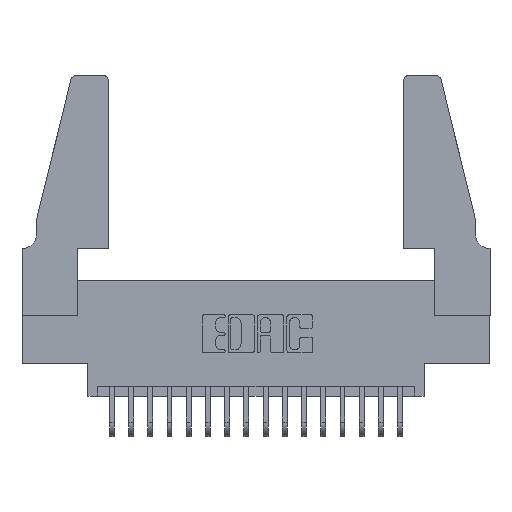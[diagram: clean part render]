
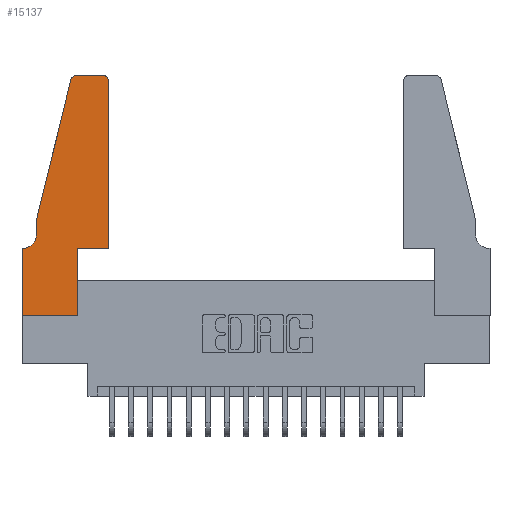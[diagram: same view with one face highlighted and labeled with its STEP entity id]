
A CAD part, top view. The second image highlights one B-rep face of the part: STEP entity #15137.
In plain terms, the highlighted planar face has unit normal (0, 0, 1).
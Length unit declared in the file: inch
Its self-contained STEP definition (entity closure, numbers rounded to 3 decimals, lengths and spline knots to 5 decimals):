
#219 = DIRECTION ( 'NONE',  ( 0., 0., 1. ) ) ;
#466 = EDGE_LOOP ( 'NONE', ( #16806, #18233, #15224, #2376, #16468, #2192, #2934, #1054, #9413, #13160, #19247, #13329 ) ) ;
#590 = VERTEX_POINT ( 'NONE', #2624 ) ;
#904 = AXIS2_PLACEMENT_3D ( 'NONE', #11156, #1846, #12693 ) ;
#1036 = DIRECTION ( 'NONE',  ( -0.239, -0.971, 0. ) ) ;
#1054 = ORIENTED_EDGE ( 'NONE', *, *, #2095, .T. ) ;
#1112 = EDGE_CURVE ( 'NONE', #2740, #590, #12800, .T. ) ;
#1832 = VERTEX_POINT ( 'NONE', #8093 ) ;
#1846 = DIRECTION ( 'NONE',  ( 0., 0., 1. ) ) ;
#1864 = LINE ( 'NONE', #18925, #17816 ) ;
#1996 = CARTESIAN_POINT ( 'NONE',  ( 0.0055, 0.42, 0.37 ) ) ;
#2095 = EDGE_CURVE ( 'NONE', #8493, #2740, #3564, .T. ) ;
#2192 = ORIENTED_EDGE ( 'NONE', *, *, #6867, .T. ) ;
#2376 = ORIENTED_EDGE ( 'NONE', *, *, #12319, .T. ) ;
#2624 = CARTESIAN_POINT ( 'NONE',  ( 0.2865, 0.35, 0.37 ) ) ;
#2740 = VERTEX_POINT ( 'NONE', #13119 ) ;
#2934 = ORIENTED_EDGE ( 'NONE', *, *, #7470, .T. ) ;
#3076 = CARTESIAN_POINT ( 'NONE',  ( 0.0755, 0.5, 0.37 ) ) ;
#3233 = DIRECTION ( 'NONE',  ( 0., 1., 0. ) ) ;
#3564 = LINE ( 'NONE', #8629, #16355 ) ;
#3566 = DIRECTION ( 'NONE',  ( -1., 0., 0. ) ) ;
#3682 = CARTESIAN_POINT ( 'NONE',  ( 0.0755, 0.35, 0.37 ) ) ;
#4038 = VERTEX_POINT ( 'NONE', #10125 ) ;
#4197 = CARTESIAN_POINT ( 'NONE',  ( 0.0755, 0.5, 0.37 ) ) ;
#4335 = CARTESIAN_POINT ( 'NONE',  ( 0., 0., 0.37 ) ) ;
#5268 = DIRECTION ( 'NONE',  ( -1., 0., 0. ) ) ;
#5428 = AXIS2_PLACEMENT_3D ( 'NONE', #6607, #17380, #8152 ) ;
#5600 = VECTOR ( 'NONE', #6764, 39.37008 ) ;
#5703 = VECTOR ( 'NONE', #7060, 39.37008 ) ;
#6096 = LINE ( 'NONE', #19104, #5600 ) ;
#6125 = EDGE_CURVE ( 'NONE', #7787, #16959, #12866, .T. ) ;
#6607 = CARTESIAN_POINT ( 'NONE',  ( 0.4205, 1.22, 0.37 ) ) ;
#6764 = DIRECTION ( 'NONE',  ( 0., 1., 0. ) ) ;
#6867 = EDGE_CURVE ( 'NONE', #16959, #18487, #9449, .T. ) ;
#7060 = DIRECTION ( 'NONE',  ( -1., 0., 0. ) ) ;
#7470 = EDGE_CURVE ( 'NONE', #18487, #8493, #1864, .T. ) ;
#7595 = CARTESIAN_POINT ( 'NONE',  ( 0.4505, 0.35, 0.37 ) ) ;
#7738 = LINE ( 'NONE', #16715, #11854 ) ;
#7787 = VERTEX_POINT ( 'NONE', #16619 ) ;
#8093 = CARTESIAN_POINT ( 'NONE',  ( 0.4205, 1.25, 0.37 ) ) ;
#8152 = DIRECTION ( 'NONE',  ( 1., 0., 0. ) ) ;
#8429 = EDGE_CURVE ( 'NONE', #13357, #12403, #13708, .T. ) ;
#8493 = VERTEX_POINT ( 'NONE', #4335 ) ;
#8629 = CARTESIAN_POINT ( 'NONE',  ( 0., 0., 0.37 ) ) ;
#9413 = ORIENTED_EDGE ( 'NONE', *, *, #1112, .T. ) ;
#9449 = LINE ( 'NONE', #3682, #9927 ) ;
#9527 = EDGE_CURVE ( 'NONE', #1832, #12207, #10296, .T. ) ;
#9563 = CIRCLE ( 'NONE', #5428, 0.03 ) ;
#9927 = VECTOR ( 'NONE', #5268, 39.37008 ) ;
#10018 = CARTESIAN_POINT ( 'NONE',  ( 0.4505, 0.35, 0.37 ) ) ;
#10125 = CARTESIAN_POINT ( 'NONE',  ( 0.4505, 1.22, 0.37 ) ) ;
#10186 = CARTESIAN_POINT ( 'NONE',  ( 0.2605, 1.25, 0.37 ) ) ;
#10203 = DIRECTION ( 'NONE',  ( 1., 0., 0. ) ) ;
#10296 = LINE ( 'NONE', #10186, #5703 ) ;
#11008 = CARTESIAN_POINT ( 'NONE',  ( 0., 0.35, 0.37 ) ) ;
#11072 = DIRECTION ( 'NONE',  ( 1., 0., 0. ) ) ;
#11156 = CARTESIAN_POINT ( 'NONE',  ( 0.284, 1.22, 0.37 ) ) ;
#11550 = DIRECTION ( 'NONE',  ( 1., 0., 0. ) ) ;
#11854 = VECTOR ( 'NONE', #18319, 39.37008 ) ;
#12122 = FACE_OUTER_BOUND ( 'NONE', #466, .T. ) ;
#12207 = VERTEX_POINT ( 'NONE', #13417 ) ;
#12319 = EDGE_CURVE ( 'NONE', #12403, #7787, #7738, .T. ) ;
#12325 = VECTOR ( 'NONE', #3233, 39.37008 ) ;
#12341 = CARTESIAN_POINT ( 'NONE',  ( 0., 0.35, 0.37 ) ) ;
#12403 = VERTEX_POINT ( 'NONE', #3076 ) ;
#12693 = DIRECTION ( 'NONE',  ( 1., 0., 0. ) ) ;
#12800 = LINE ( 'NONE', #14103, #12325 ) ;
#12802 = DIRECTION ( 'NONE',  ( 0., -1., 0. ) ) ;
#12834 = DIRECTION ( 'NONE',  ( 0., 0., -1. ) ) ;
#12866 = CIRCLE ( 'NONE', #18377, 0.07 ) ;
#13119 = CARTESIAN_POINT ( 'NONE',  ( 0.2865, 0., 0.37 ) ) ;
#13160 = ORIENTED_EDGE ( 'NONE', *, *, #19455, .T. ) ;
#13221 = EDGE_CURVE ( 'NONE', #4038, #1832, #9563, .T. ) ;
#13329 = ORIENTED_EDGE ( 'NONE', *, *, #13221, .T. ) ;
#13357 = VERTEX_POINT ( 'NONE', #19198 ) ;
#13417 = CARTESIAN_POINT ( 'NONE',  ( 0.284, 1.25, 0.37 ) ) ;
#13458 = AXIS2_PLACEMENT_3D ( 'NONE', #11008, #219, #11072 ) ;
#13708 = LINE ( 'NONE', #4197, #17783 ) ;
#13949 = CIRCLE ( 'NONE', #904, 0.03 ) ;
#14103 = CARTESIAN_POINT ( 'NONE',  ( 0.2865, 0.35, 0.37 ) ) ;
#15137 = ADVANCED_FACE ( 'NONE', ( #12122 ), #17186, .T. ) ;
#15224 = ORIENTED_EDGE ( 'NONE', *, *, #8429, .T. ) ;
#15598 = VECTOR ( 'NONE', #11550, 39.37008 ) ;
#15983 = EDGE_CURVE ( 'NONE', #16582, #4038, #6096, .T. ) ;
#16355 = VECTOR ( 'NONE', #10203, 39.37008 ) ;
#16468 = ORIENTED_EDGE ( 'NONE', *, *, #6125, .T. ) ;
#16582 = VERTEX_POINT ( 'NONE', #7595 ) ;
#16619 = CARTESIAN_POINT ( 'NONE',  ( 0.0755, 0.42, 0.37 ) ) ;
#16715 = CARTESIAN_POINT ( 'NONE',  ( 0.0755, 0.5, 0.37 ) ) ;
#16806 = ORIENTED_EDGE ( 'NONE', *, *, #9527, .T. ) ;
#16959 = VERTEX_POINT ( 'NONE', #17691 ) ;
#17034 = LINE ( 'NONE', #10018, #15598 ) ;
#17186 = PLANE ( 'NONE',  #13458 ) ;
#17380 = DIRECTION ( 'NONE',  ( 0., 0., 1. ) ) ;
#17691 = CARTESIAN_POINT ( 'NONE',  ( 0.0055, 0.35, 0.37 ) ) ;
#17783 = VECTOR ( 'NONE', #1036, 39.37008 ) ;
#17816 = VECTOR ( 'NONE', #12802, 39.37008 ) ;
#17963 = EDGE_CURVE ( 'NONE', #12207, #13357, #13949, .T. ) ;
#18233 = ORIENTED_EDGE ( 'NONE', *, *, #17963, .T. ) ;
#18319 = DIRECTION ( 'NONE',  ( 0., -1., 0. ) ) ;
#18377 = AXIS2_PLACEMENT_3D ( 'NONE', #1996, #12834, #3566 ) ;
#18487 = VERTEX_POINT ( 'NONE', #12341 ) ;
#18925 = CARTESIAN_POINT ( 'NONE',  ( 0., 0., 0.37 ) ) ;
#19104 = CARTESIAN_POINT ( 'NONE',  ( 0.4505, 0.35, 0.37 ) ) ;
#19198 = CARTESIAN_POINT ( 'NONE',  ( 0.25487, 1.22718, 0.37 ) ) ;
#19247 = ORIENTED_EDGE ( 'NONE', *, *, #15983, .T. ) ;
#19455 = EDGE_CURVE ( 'NONE', #590, #16582, #17034, .T. ) ;
